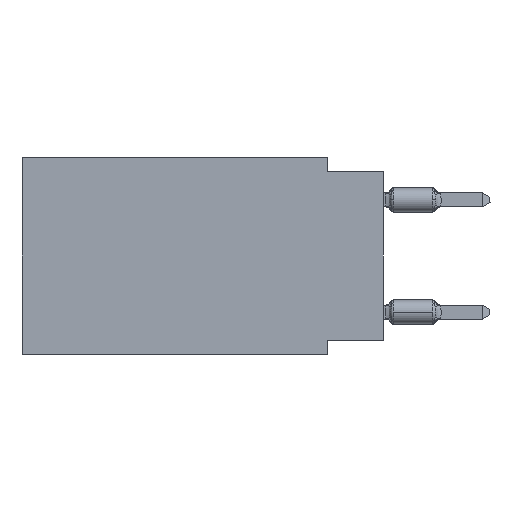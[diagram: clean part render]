
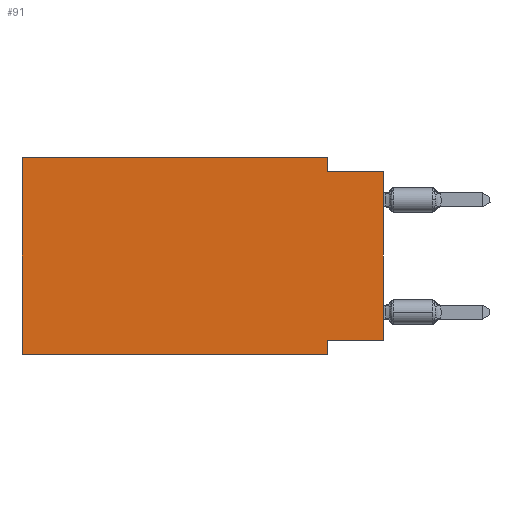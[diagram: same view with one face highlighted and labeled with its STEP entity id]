
A CAD part, left-side view. The second image highlights one B-rep face of the part: STEP entity #91.
In plain terms, the highlighted planar face has unit normal (-1, 0, 0).
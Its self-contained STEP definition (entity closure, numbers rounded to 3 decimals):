
#91 = ADVANCED_FACE ( 'NONE', ( #12657 ), #10941, .F. ) ;
#671 = VECTOR ( 'NONE', #9854, 1000. ) ;
#1008 = ORIENTED_EDGE ( 'NONE', *, *, #26194, .F. ) ;
#1173 = EDGE_CURVE ( 'NONE', #8580, #26780, #9017, .T. ) ;
#1538 = VERTEX_POINT ( 'NONE', #14359 ) ;
#1694 = DIRECTION ( 'NONE',  ( 0., 0., -1. ) ) ;
#2188 = ORIENTED_EDGE ( 'NONE', *, *, #7240, .F. ) ;
#2200 = CARTESIAN_POINT ( 'NONE',  ( 0., 16.383, 0. ) ) ;
#2267 = CARTESIAN_POINT ( 'NONE',  ( 0., 16.383, 0. ) ) ;
#2591 = CARTESIAN_POINT ( 'NONE',  ( 0., 0., -0.635 ) ) ;
#3925 = VECTOR ( 'NONE', #4871, 1000. ) ;
#4871 = DIRECTION ( 'NONE',  ( 0., -1., 0. ) ) ;
#5035 = DIRECTION ( 'NONE',  ( 0., 0., -1. ) ) ;
#5100 = EDGE_CURVE ( 'NONE', #14060, #16956, #22839, .T. ) ;
#5162 = EDGE_CURVE ( 'NONE', #14060, #24559, #24217, .T. ) ;
#5406 = ORIENTED_EDGE ( 'NONE', *, *, #16243, .T. ) ;
#5735 = ORIENTED_EDGE ( 'NONE', *, *, #1173, .F. ) ;
#7240 = EDGE_CURVE ( 'NONE', #14713, #8580, #16192, .T. ) ;
#8055 = ORIENTED_EDGE ( 'NONE', *, *, #5162, .F. ) ;
#8476 = VECTOR ( 'NONE', #11541, 1000. ) ;
#8580 = VERTEX_POINT ( 'NONE', #8626 ) ;
#8626 = CARTESIAN_POINT ( 'NONE',  ( 0., 16.383, 0. ) ) ;
#9017 = LINE ( 'NONE', #2200, #19190 ) ;
#9071 = EDGE_LOOP ( 'NONE', ( #23244, #1008, #17527, #5735, #2188, #5406, #18991, #8055 ) ) ;
#9675 = LINE ( 'NONE', #20099, #8476 ) ;
#9767 = CARTESIAN_POINT ( 'NONE',  ( 0., 16.383, 0. ) ) ;
#9854 = DIRECTION ( 'NONE',  ( 0., 0., 1. ) ) ;
#10838 = VECTOR ( 'NONE', #20622, 1000. ) ;
#10875 = DIRECTION ( 'NONE',  ( 0., -1., 0. ) ) ;
#10941 = PLANE ( 'NONE',  #20553 ) ;
#11541 = DIRECTION ( 'NONE',  ( 0., 0., -1. ) ) ;
#11552 = LINE ( 'NONE', #26950, #3925 ) ;
#11571 = CARTESIAN_POINT ( 'NONE',  ( 0., 2.54, 0. ) ) ;
#11581 = VECTOR ( 'NONE', #21395, 1000. ) ;
#11662 = CARTESIAN_POINT ( 'NONE',  ( 0., 2.54, 0. ) ) ;
#12657 = FACE_OUTER_BOUND ( 'NONE', #9071, .T. ) ;
#12695 = VECTOR ( 'NONE', #5035, 1000. ) ;
#13228 = DIRECTION ( 'NONE',  ( 1., 0., 0. ) ) ;
#14060 = VERTEX_POINT ( 'NONE', #18456 ) ;
#14359 = CARTESIAN_POINT ( 'NONE',  ( 0., 2.54, -0.635 ) ) ;
#14713 = VERTEX_POINT ( 'NONE', #25922 ) ;
#16192 = LINE ( 'NONE', #9767, #10838 ) ;
#16243 = EDGE_CURVE ( 'NONE', #14713, #23598, #11552, .T. ) ;
#16956 = VERTEX_POINT ( 'NONE', #24999 ) ;
#17527 = ORIENTED_EDGE ( 'NONE', *, *, #22342, .F. ) ;
#18456 = CARTESIAN_POINT ( 'NONE',  ( 0., 0., -8.255 ) ) ;
#18966 = CARTESIAN_POINT ( 'NONE',  ( 0., 2.54, -8.89 ) ) ;
#18991 = ORIENTED_EDGE ( 'NONE', *, *, #23870, .F. ) ;
#19190 = VECTOR ( 'NONE', #10875, 1000. ) ;
#20099 = CARTESIAN_POINT ( 'NONE',  ( 0., 2.54, -8.89 ) ) ;
#20553 = AXIS2_PLACEMENT_3D ( 'NONE', #2267, #13228, #1694 ) ;
#20622 = DIRECTION ( 'NONE',  ( 0., 0., 1. ) ) ;
#20706 = CARTESIAN_POINT ( 'NONE',  ( 0., 0., 0. ) ) ;
#21395 = DIRECTION ( 'NONE',  ( 0., 1., 0. ) ) ;
#22342 = EDGE_CURVE ( 'NONE', #26780, #1538, #24839, .T. ) ;
#22384 = LINE ( 'NONE', #2591, #26385 ) ;
#22839 = LINE ( 'NONE', #20706, #671 ) ;
#23244 = ORIENTED_EDGE ( 'NONE', *, *, #5100, .T. ) ;
#23598 = VERTEX_POINT ( 'NONE', #18966 ) ;
#23870 = EDGE_CURVE ( 'NONE', #24559, #23598, #9675, .T. ) ;
#23885 = CARTESIAN_POINT ( 'NONE',  ( 0., 2.54, -8.255 ) ) ;
#24067 = CARTESIAN_POINT ( 'NONE',  ( 0., 0., -8.255 ) ) ;
#24217 = LINE ( 'NONE', #24067, #11581 ) ;
#24559 = VERTEX_POINT ( 'NONE', #23885 ) ;
#24839 = LINE ( 'NONE', #11571, #12695 ) ;
#24999 = CARTESIAN_POINT ( 'NONE',  ( 0., 0., -0.635 ) ) ;
#25922 = CARTESIAN_POINT ( 'NONE',  ( 0., 16.383, -8.89 ) ) ;
#26194 = EDGE_CURVE ( 'NONE', #1538, #16956, #22384, .T. ) ;
#26385 = VECTOR ( 'NONE', #26668, 1000. ) ;
#26668 = DIRECTION ( 'NONE',  ( 0., -1., 0. ) ) ;
#26780 = VERTEX_POINT ( 'NONE', #11662 ) ;
#26950 = CARTESIAN_POINT ( 'NONE',  ( 0., 16.383, -8.89 ) ) ;
